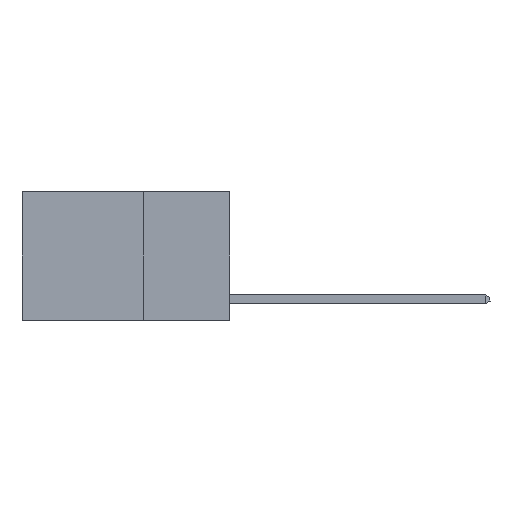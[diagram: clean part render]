
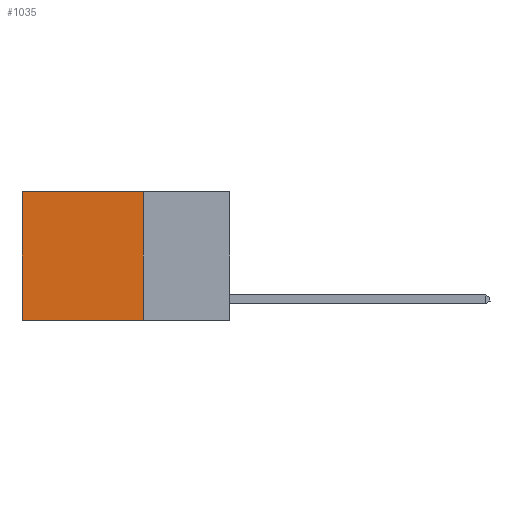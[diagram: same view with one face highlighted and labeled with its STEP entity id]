
A CAD part, left-side view. The second image highlights one B-rep face of the part: STEP entity #1035.
In plain terms, the highlighted planar face has unit normal (-1, 0, 0).
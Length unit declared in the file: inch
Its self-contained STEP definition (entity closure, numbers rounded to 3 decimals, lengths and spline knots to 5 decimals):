
#213 = LINE ( 'NONE', #13511, #8037 ) ;
#451 = EDGE_CURVE ( 'NONE', #9807, #6686, #12531, .T. ) ;
#529 = DIRECTION ( 'NONE',  ( 0., 1., 0. ) ) ;
#682 = EDGE_CURVE ( 'NONE', #12743, #14330, #4580, .T. ) ;
#707 = CARTESIAN_POINT ( 'NONE',  ( 0.2625, 0.25, 0. ) ) ;
#1035 = ADVANCED_FACE ( 'NONE', ( #9513 ), #9165, .F. ) ;
#1168 = DIRECTION ( 'NONE',  ( 0., 0., -1. ) ) ;
#1729 = VECTOR ( 'NONE', #529, 39.37008 ) ;
#1890 = VECTOR ( 'NONE', #10917, 39.37008 ) ;
#2330 = DIRECTION ( 'NONE',  ( 1., 0., 0. ) ) ;
#3425 = VECTOR ( 'NONE', #4376, 39.37008 ) ;
#4376 = DIRECTION ( 'NONE',  ( 0., 0., -1. ) ) ;
#4580 = LINE ( 'NONE', #707, #1890 ) ;
#5520 = CARTESIAN_POINT ( 'NONE',  ( 0.2625, 0.25, 0. ) ) ;
#5527 = EDGE_LOOP ( 'NONE', ( #7871, #13264, #11153, #6633 ) ) ;
#5924 = EDGE_CURVE ( 'NONE', #12743, #9807, #13661, .T. ) ;
#6628 = CARTESIAN_POINT ( 'NONE',  ( 0.2625, 0.25, -0.37 ) ) ;
#6633 = ORIENTED_EDGE ( 'NONE', *, *, #682, .T. ) ;
#6686 = VERTEX_POINT ( 'NONE', #13117 ) ;
#7622 = CARTESIAN_POINT ( 'NONE',  ( 0.2625, 0.25, 0. ) ) ;
#7871 = ORIENTED_EDGE ( 'NONE', *, *, #13096, .T. ) ;
#8037 = VECTOR ( 'NONE', #1168, 39.37008 ) ;
#9165 = PLANE ( 'NONE',  #9444 ) ;
#9267 = CARTESIAN_POINT ( 'NONE',  ( 0.2625, 0.6, 0. ) ) ;
#9444 = AXIS2_PLACEMENT_3D ( 'NONE', #12608, #2330, #13720 ) ;
#9513 = FACE_OUTER_BOUND ( 'NONE', #5527, .T. ) ;
#9807 = VERTEX_POINT ( 'NONE', #6628 ) ;
#10917 = DIRECTION ( 'NONE',  ( 0., 1., 0. ) ) ;
#11153 = ORIENTED_EDGE ( 'NONE', *, *, #5924, .F. ) ;
#12531 = LINE ( 'NONE', #14056, #1729 ) ;
#12608 = CARTESIAN_POINT ( 'NONE',  ( 0.2625, 0.25, 0. ) ) ;
#12743 = VERTEX_POINT ( 'NONE', #7622 ) ;
#13096 = EDGE_CURVE ( 'NONE', #14330, #6686, #213, .T. ) ;
#13117 = CARTESIAN_POINT ( 'NONE',  ( 0.2625, 0.6, -0.37 ) ) ;
#13264 = ORIENTED_EDGE ( 'NONE', *, *, #451, .F. ) ;
#13511 = CARTESIAN_POINT ( 'NONE',  ( 0.2625, 0.6, 0. ) ) ;
#13661 = LINE ( 'NONE', #5520, #3425 ) ;
#13720 = DIRECTION ( 'NONE',  ( 0., 0., -1. ) ) ;
#14056 = CARTESIAN_POINT ( 'NONE',  ( 0.2625, 0.25, -0.37 ) ) ;
#14330 = VERTEX_POINT ( 'NONE', #9267 ) ;
